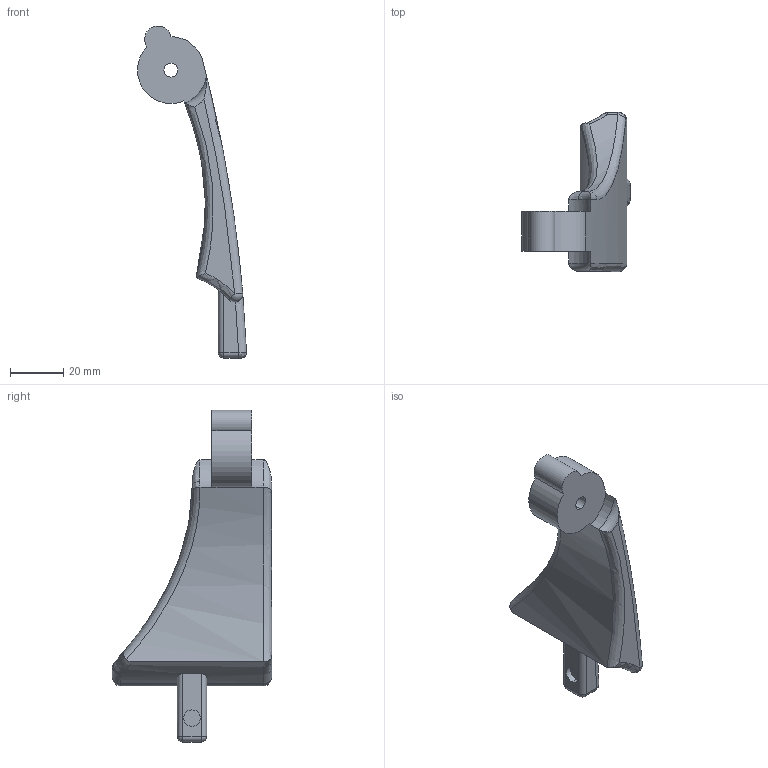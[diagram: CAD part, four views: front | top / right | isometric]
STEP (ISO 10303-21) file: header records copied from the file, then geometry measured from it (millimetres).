
FILE_DESCRIPTION (( 'STEP AP203' ), '1' );
FILE_NAME ('ArmL.STEP', '2020-10-24T03:16:24', ( '' ), ( '' ), 'SwSTEP 2.0', 'SolidWorks 2019', '' );
FILE_SCHEMA (( 'CONFIG_CONTROL_DESIGN' ));
Length unit declared in the file: millimetre
Products named in the file (1): ArmL
Bounding box: 41.08 x 60 x 125.12 mm (x, y, z)
Volume: 45526 mm3; surface area: 12104.1 mm2
Topology: 1 solids, 1 shells, 58 faces, 145 edges, 84 vertices
Faces by surface type: cylinder 23, bspline 15, plane 10, sphere 6, torus 4
Entity records: 2526 total; most frequent: CARTESIAN_POINT 1208, ORIENTED_EDGE 278, DIRECTION 235, EDGE_CURVE 139, AXIS2_PLACEMENT_3D 99, VERTEX_POINT 84, EDGE_LOOP 61, ADVANCED_FACE 58
